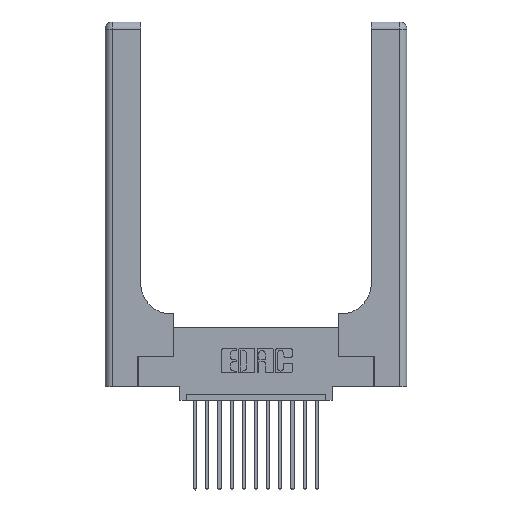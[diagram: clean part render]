
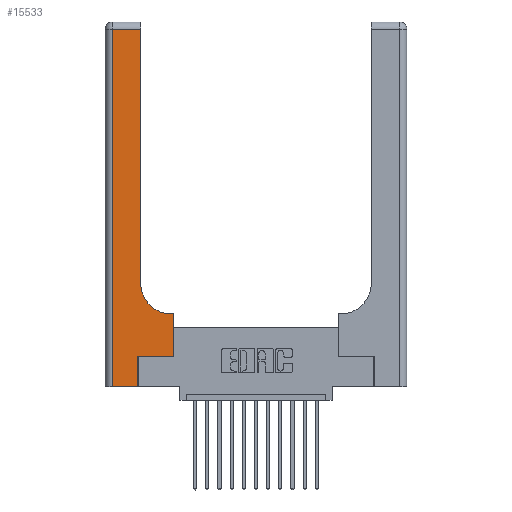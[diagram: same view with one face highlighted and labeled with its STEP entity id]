
A CAD part, top view. The second image highlights one B-rep face of the part: STEP entity #15533.
In plain terms, the highlighted planar face has unit normal (0, 0, 1).
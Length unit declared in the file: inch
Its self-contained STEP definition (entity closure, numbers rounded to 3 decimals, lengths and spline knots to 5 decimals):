
#319 = LINE ( 'NONE', #4491, #17092 ) ;
#882 = DIRECTION ( 'NONE',  ( -1., 0., 0. ) ) ;
#1084 = FACE_OUTER_BOUND ( 'NONE', #14189, .T. ) ;
#1208 = VERTEX_POINT ( 'NONE', #10840 ) ;
#1813 = DIRECTION ( 'NONE',  ( 0., 1., 0. ) ) ;
#1872 = CARTESIAN_POINT ( 'NONE',  ( 0.06, 0., 0.37 ) ) ;
#2314 = EDGE_CURVE ( 'NONE', #13129, #11072, #5964, .T. ) ;
#2630 = LINE ( 'NONE', #8644, #11223 ) ;
#2686 = CARTESIAN_POINT ( 'NONE',  ( 0.269, 0., 0.37 ) ) ;
#2817 = PLANE ( 'NONE',  #4673 ) ;
#3388 = DIRECTION ( 'NONE',  ( 1., 0., 0. ) ) ;
#3592 = EDGE_CURVE ( 'NONE', #14840, #13129, #319, .T. ) ;
#3794 = ORIENTED_EDGE ( 'NONE', *, *, #17585, .T. ) ;
#3838 = DIRECTION ( 'NONE',  ( 1., 0., 0. ) ) ;
#4137 = CARTESIAN_POINT ( 'NONE',  ( 0.2915, 0.85, 0.37 ) ) ;
#4491 = CARTESIAN_POINT ( 'NONE',  ( 0.06, 3., 0.37 ) ) ;
#4673 = AXIS2_PLACEMENT_3D ( 'NONE', #9469, #9642, #8209 ) ;
#4812 = CIRCLE ( 'NONE', #17210, 0.25 ) ;
#4825 = LINE ( 'NONE', #8774, #7581 ) ;
#5146 = VECTOR ( 'NONE', #13280, 39.37008 ) ;
#5311 = CARTESIAN_POINT ( 'NONE',  ( 0.5415, 0.85, 0.37 ) ) ;
#5359 = ORIENTED_EDGE ( 'NONE', *, *, #17666, .T. ) ;
#5428 = VERTEX_POINT ( 'NONE', #7612 ) ;
#5470 = EDGE_CURVE ( 'NONE', #5428, #5501, #4812, .T. ) ;
#5501 = VERTEX_POINT ( 'NONE', #4137 ) ;
#5947 = CARTESIAN_POINT ( 'NONE',  ( 0., 2.94, 0.37 ) ) ;
#5964 = LINE ( 'NONE', #17558, #5146 ) ;
#6046 = CARTESIAN_POINT ( 'NONE',  ( 0.2915, 0.6, 0.37 ) ) ;
#6291 = VECTOR ( 'NONE', #14178, 39.37008 ) ;
#6417 = DIRECTION ( 'NONE',  ( 0., 0., -1. ) ) ;
#6692 = ORIENTED_EDGE ( 'NONE', *, *, #8312, .T. ) ;
#6871 = EDGE_CURVE ( 'NONE', #11072, #15293, #17180, .T. ) ;
#7255 = DIRECTION ( 'NONE',  ( 0., 1., 0. ) ) ;
#7581 = VECTOR ( 'NONE', #3388, 39.37008 ) ;
#7612 = CARTESIAN_POINT ( 'NONE',  ( 0.5415, 0.6, 0.37 ) ) ;
#7911 = LINE ( 'NONE', #6046, #17580 ) ;
#8209 = DIRECTION ( 'NONE',  ( -1., 0., 0. ) ) ;
#8312 = EDGE_CURVE ( 'NONE', #9457, #5428, #7911, .T. ) ;
#8644 = CARTESIAN_POINT ( 'NONE',  ( 0.2915, 3., 0.37 ) ) ;
#8774 = CARTESIAN_POINT ( 'NONE',  ( 0.269, 0.25, 0.37 ) ) ;
#9078 = ORIENTED_EDGE ( 'NONE', *, *, #13613, .T. ) ;
#9457 = VERTEX_POINT ( 'NONE', #15270 ) ;
#9469 = CARTESIAN_POINT ( 'NONE',  ( 0., 3., 0.37 ) ) ;
#9591 = ORIENTED_EDGE ( 'NONE', *, *, #2314, .T. ) ;
#9642 = DIRECTION ( 'NONE',  ( 0., 0., -1. ) ) ;
#9724 = ORIENTED_EDGE ( 'NONE', *, *, #5470, .T. ) ;
#10072 = VECTOR ( 'NONE', #16723, 39.37008 ) ;
#10219 = CARTESIAN_POINT ( 'NONE',  ( 0.5585, 0.25, 0.37 ) ) ;
#10251 = ORIENTED_EDGE ( 'NONE', *, *, #6871, .T. ) ;
#10331 = ORIENTED_EDGE ( 'NONE', *, *, #3592, .T. ) ;
#10410 = CARTESIAN_POINT ( 'NONE',  ( 0.269, 0.25, 0.37 ) ) ;
#10840 = CARTESIAN_POINT ( 'NONE',  ( 0.2915, 2.94, 0.37 ) ) ;
#11072 = VERTEX_POINT ( 'NONE', #2686 ) ;
#11223 = VECTOR ( 'NONE', #1813, 39.37008 ) ;
#12838 = DIRECTION ( 'NONE',  ( 0., -1., 0. ) ) ;
#13129 = VERTEX_POINT ( 'NONE', #1872 ) ;
#13186 = VECTOR ( 'NONE', #7255, 39.37008 ) ;
#13280 = DIRECTION ( 'NONE',  ( 1., 0., 0. ) ) ;
#13390 = LINE ( 'NONE', #5947, #6291 ) ;
#13613 = EDGE_CURVE ( 'NONE', #5501, #1208, #2630, .T. ) ;
#13754 = CARTESIAN_POINT ( 'NONE',  ( 0.5585, 0.25, 0.37 ) ) ;
#14088 = CARTESIAN_POINT ( 'NONE',  ( 0.269, 0., 0.37 ) ) ;
#14178 = DIRECTION ( 'NONE',  ( -1., 0., 0. ) ) ;
#14189 = EDGE_LOOP ( 'NONE', ( #9078, #3794, #10331, #9591, #10251, #17440, #5359, #6692, #9724 ) ) ;
#14840 = VERTEX_POINT ( 'NONE', #17377 ) ;
#15146 = VERTEX_POINT ( 'NONE', #10219 ) ;
#15270 = CARTESIAN_POINT ( 'NONE',  ( 0.5585, 0.6, 0.37 ) ) ;
#15293 = VERTEX_POINT ( 'NONE', #10410 ) ;
#15533 = ADVANCED_FACE ( 'NONE', ( #1084 ), #2817, .F. ) ;
#16690 = EDGE_CURVE ( 'NONE', #15293, #15146, #4825, .T. ) ;
#16723 = DIRECTION ( 'NONE',  ( 0., 1., 0. ) ) ;
#16799 = LINE ( 'NONE', #13754, #13186 ) ;
#17092 = VECTOR ( 'NONE', #12838, 39.37008 ) ;
#17180 = LINE ( 'NONE', #14088, #10072 ) ;
#17210 = AXIS2_PLACEMENT_3D ( 'NONE', #5311, #6417, #3838 ) ;
#17377 = CARTESIAN_POINT ( 'NONE',  ( 0.06, 2.94, 0.37 ) ) ;
#17440 = ORIENTED_EDGE ( 'NONE', *, *, #16690, .T. ) ;
#17558 = CARTESIAN_POINT ( 'NONE',  ( 0., 0., 0.37 ) ) ;
#17580 = VECTOR ( 'NONE', #882, 39.37008 ) ;
#17585 = EDGE_CURVE ( 'NONE', #1208, #14840, #13390, .T. ) ;
#17666 = EDGE_CURVE ( 'NONE', #15146, #9457, #16799, .T. ) ;
